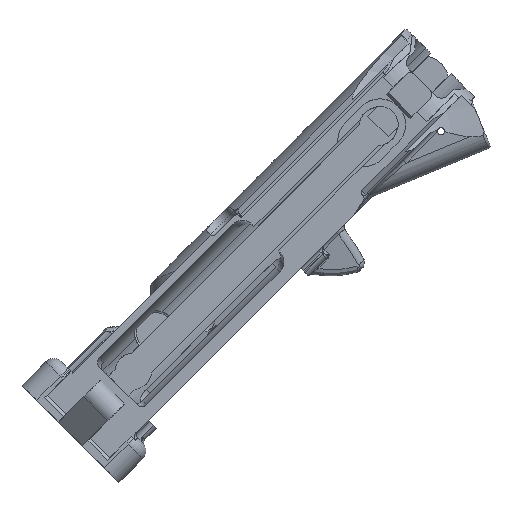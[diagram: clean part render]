
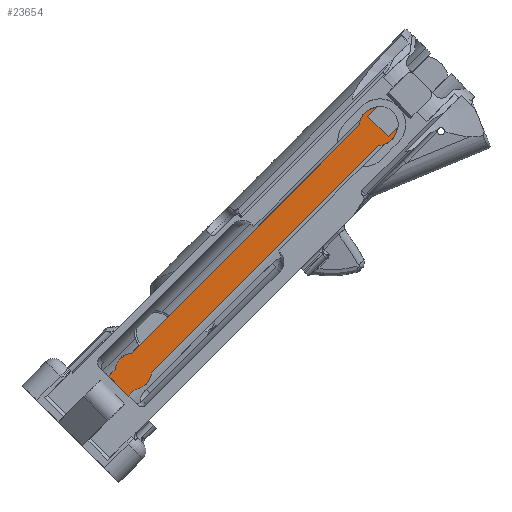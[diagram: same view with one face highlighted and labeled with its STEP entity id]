
A CAD part, top view. The second image highlights one B-rep face of the part: STEP entity #23654.
In plain terms, the highlighted planar face has unit normal (0, 0, 1).
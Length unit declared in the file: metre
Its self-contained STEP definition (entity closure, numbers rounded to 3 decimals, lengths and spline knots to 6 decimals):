
#1530=CIRCLE('',#24801,0.007087);
#1531=CIRCLE('',#24803,0.007087);
#1679=CIRCLE('',#25189,0.006769);
#1680=CIRCLE('',#25190,0.006769);
#6271=ORIENTED_EDGE('',*,*,#11632,.F.);
#6272=ORIENTED_EDGE('',*,*,#10905,.T.);
#6273=ORIENTED_EDGE('',*,*,#11633,.T.);
#6274=ORIENTED_EDGE('',*,*,#11565,.F.);
#6275=ORIENTED_EDGE('',*,*,#11634,.F.);
#6276=ORIENTED_EDGE('',*,*,#10900,.T.);
#6277=ORIENTED_EDGE('',*,*,#11635,.F.);
#6278=ORIENTED_EDGE('',*,*,#11636,.T.);
#6279=ORIENTED_EDGE('',*,*,#11144,.T.);
#6280=ORIENTED_EDGE('',*,*,#11139,.T.);
#6281=ORIENTED_EDGE('',*,*,#11148,.T.);
#6282=ORIENTED_EDGE('',*,*,#11637,.T.);
#10900=EDGE_CURVE('',#13818,#13817,#1530,.T.);
#10905=EDGE_CURVE('',#13823,#13822,#1531,.T.);
#11139=EDGE_CURVE('',#13974,#13973,#16221,.T.);
#11144=EDGE_CURVE('',#13976,#13974,#16226,.T.);
#11148=EDGE_CURVE('',#13973,#13980,#16230,.T.);
#11565=EDGE_CURVE('',#14268,#14269,#16577,.T.);
#11632=EDGE_CURVE('',#13823,#14300,#16619,.T.);
#11633=EDGE_CURVE('',#13822,#14269,#16620,.T.);
#11634=EDGE_CURVE('',#13818,#14268,#16621,.T.);
#11635=EDGE_CURVE('',#14301,#13817,#16622,.T.);
#11636=EDGE_CURVE('',#14301,#13976,#1679,.F.);
#11637=EDGE_CURVE('',#13980,#14300,#1680,.F.);
#13817=VERTEX_POINT('',#37750);
#13818=VERTEX_POINT('',#37752);
#13822=VERTEX_POINT('',#37767);
#13823=VERTEX_POINT('',#37769);
#13973=VERTEX_POINT('',#39273);
#13974=VERTEX_POINT('',#39275);
#13976=VERTEX_POINT('',#39280);
#13980=VERTEX_POINT('',#39291);
#14268=VERTEX_POINT('',#40184);
#14269=VERTEX_POINT('',#40186);
#14300=VERTEX_POINT('',#40426);
#14301=VERTEX_POINT('',#40430);
#16221=LINE('',#39274,#18576);
#16226=LINE('',#39284,#18581);
#16230=LINE('',#39292,#18585);
#16577=LINE('',#40185,#18932);
#16619=LINE('',#40425,#18974);
#16620=LINE('',#40427,#18975);
#16621=LINE('',#40428,#18976);
#16622=LINE('',#40429,#18977);
#18576=VECTOR('',#28857,1.);
#18581=VECTOR('',#28864,1.);
#18585=VECTOR('',#28870,1.);
#18932=VECTOR('',#29569,1.);
#18974=VECTOR('',#29701,1.);
#18975=VECTOR('',#29702,1.);
#18976=VECTOR('',#29703,1.);
#18977=VECTOR('',#29704,1.);
#20234=EDGE_LOOP('',(#6271,#6272,#6273,#6274,#6275,#6276,#6277,#6278,#6279,
#6280,#6281,#6282));
#21595=FACE_BOUND('',#20234,.T.);
#22640=PLANE('',#25188);
#23654=ADVANCED_FACE('',(#21595),#22640,.F.);
#24801=AXIS2_PLACEMENT_3D('',#37751,#28429,#28430);
#24803=AXIS2_PLACEMENT_3D('',#37768,#28436,#28437);
#25188=AXIS2_PLACEMENT_3D('',#40424,#29699,#29700);
#25189=AXIS2_PLACEMENT_3D('',#40431,#29705,#29706);
#25190=AXIS2_PLACEMENT_3D('',#40432,#29707,#29708);
#28429=DIRECTION('',(0.,0.,1.));
#28430=DIRECTION('',(-0.707,0.707,0.));
#28436=DIRECTION('',(0.,0.,1.));
#28437=DIRECTION('',(-0.707,0.707,0.));
#28857=DIRECTION('',(0.707,-0.707,0.));
#28864=DIRECTION('',(-0.707,-0.707,0.));
#28870=DIRECTION('',(0.707,0.707,0.));
#29569=DIRECTION('',(0.707,-0.707,0.));
#29699=DIRECTION('',(0.,0.,-1.));
#29700=DIRECTION('',(0.707,0.707,0.));
#29701=DIRECTION('',(-0.707,-0.707,0.));
#29702=DIRECTION('',(-0.707,-0.707,0.));
#29703=DIRECTION('',(-0.707,-0.707,0.));
#29704=DIRECTION('',(0.707,0.707,0.));
#29705=DIRECTION('',(0.,0.,-1.));
#29706=DIRECTION('',(-0.707,0.707,0.));
#29707=DIRECTION('',(0.,0.,-1.));
#29708=DIRECTION('',(-0.707,0.707,0.));
#37750=CARTESIAN_POINT('',(0.072524,0.134174,0.005207));
#37751=CARTESIAN_POINT('',(0.079558,0.133305,0.005207));
#37752=CARTESIAN_POINT('',(0.079162,0.140381,0.005207));
#37767=CARTESIAN_POINT('',(0.086633,0.132909,0.005207));
#37768=CARTESIAN_POINT('',(0.079558,0.133305,0.005207));
#37769=CARTESIAN_POINT('',(0.080427,0.126271,0.005207));
#39273=CARTESIAN_POINT('',(-0.013029,0.033355,0.005207));
#39274=CARTESIAN_POINT('',(-0.01073,0.031056,0.005207));
#39275=CARTESIAN_POINT('',(-0.020393,0.040718,0.005207));
#39280=CARTESIAN_POINT('',(-0.017883,0.043228,0.005207));
#39284=CARTESIAN_POINT('',(-0.030361,0.03075,0.005207));
#39291=CARTESIAN_POINT('',(-0.010519,0.035864,0.005207));
#39292=CARTESIAN_POINT('',(-0.022997,0.023386,0.005207));
#40184=CARTESIAN_POINT('',(0.075822,0.137041,0.005207));
#40185=CARTESIAN_POINT('',(0.083293,0.129569,0.005207));
#40186=CARTESIAN_POINT('',(0.083293,0.129569,0.005207));
#40424=CARTESIAN_POINT('',(-0.020698,0.021087,0.005207));
#40425=CARTESIAN_POINT('',(-0.00449,0.041354,0.005207));
#40426=CARTESIAN_POINT('',(-0.00449,0.041354,0.005207));
#40427=CARTESIAN_POINT('',(-0.022943,0.023333,0.005207));
#40428=CARTESIAN_POINT('',(0.075822,0.137041,0.005207));
#40429=CARTESIAN_POINT('',(-0.012393,0.049257,0.005207));
#40430=CARTESIAN_POINT('',(-0.012393,0.049257,0.005207));
#40431=CARTESIAN_POINT('',(-0.011143,0.042604,0.005207));
#40432=CARTESIAN_POINT('',(-0.011143,0.042604,0.005207));
